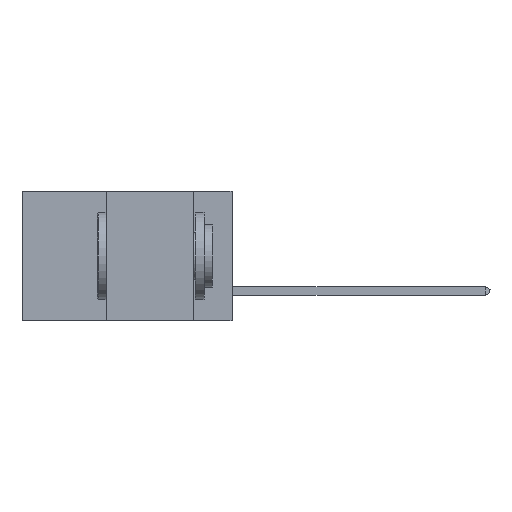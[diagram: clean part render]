
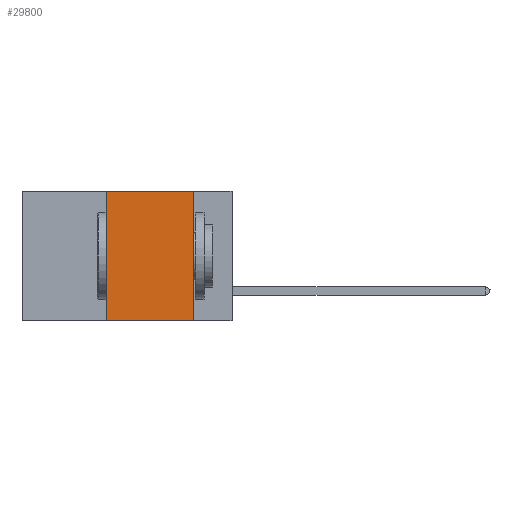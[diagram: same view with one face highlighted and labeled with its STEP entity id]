
A CAD part, left-side view. The second image highlights one B-rep face of the part: STEP entity #29800.
In plain terms, the highlighted planar face has unit normal (-1, 0, 0).
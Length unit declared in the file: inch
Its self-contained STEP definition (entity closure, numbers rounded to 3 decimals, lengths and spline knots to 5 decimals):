
#941 = LINE ( 'NONE', #6337, #48508 ) ;
#4822 = EDGE_CURVE ( 'NONE', #9141, #17668, #25303, .T. ) ;
#5923 = AXIS2_PLACEMENT_3D ( 'NONE', #14358, #9700, #25988 ) ;
#6009 = CARTESIAN_POINT ( 'NONE',  ( 0., 0.36, 0. ) ) ;
#6337 = CARTESIAN_POINT ( 'NONE',  ( 0., 0.6, -0.37 ) ) ;
#9141 = VERTEX_POINT ( 'NONE', #6009 ) ;
#9700 = DIRECTION ( 'NONE',  ( 1., 0., 0. ) ) ;
#13434 = EDGE_CURVE ( 'NONE', #17668, #29327, #38671, .T. ) ;
#14358 = CARTESIAN_POINT ( 'NONE',  ( 0., 0.6, 0. ) ) ;
#16142 = VECTOR ( 'NONE', #41430, 39.37008 ) ;
#17668 = VERTEX_POINT ( 'NONE', #37970 ) ;
#19001 = ORIENTED_EDGE ( 'NONE', *, *, #43399, .F. ) ;
#20560 = VECTOR ( 'NONE', #32418, 39.37008 ) ;
#24343 = VERTEX_POINT ( 'NONE', #46436 ) ;
#24676 = CARTESIAN_POINT ( 'NONE',  ( 0., 0.11, 0. ) ) ;
#25303 = LINE ( 'NONE', #40562, #16142 ) ;
#25525 = ORIENTED_EDGE ( 'NONE', *, *, #31946, .T. ) ;
#25988 = DIRECTION ( 'NONE',  ( 0., 0., -1. ) ) ;
#27235 = ORIENTED_EDGE ( 'NONE', *, *, #13434, .F. ) ;
#29327 = VERTEX_POINT ( 'NONE', #33696 ) ;
#29423 = DIRECTION ( 'NONE',  ( 0., -1., 0. ) ) ;
#29800 = ADVANCED_FACE ( 'NONE', ( #47466 ), #35439, .F. ) ;
#31506 = LINE ( 'NONE', #35094, #38179 ) ;
#31946 = EDGE_CURVE ( 'NONE', #24343, #29327, #941, .T. ) ;
#32418 = DIRECTION ( 'NONE',  ( 0., 0., -1. ) ) ;
#33696 = CARTESIAN_POINT ( 'NONE',  ( 0., 0.11, -0.37 ) ) ;
#35094 = CARTESIAN_POINT ( 'NONE',  ( 0., 0.36, 0. ) ) ;
#35439 = PLANE ( 'NONE',  #5923 ) ;
#37970 = CARTESIAN_POINT ( 'NONE',  ( 0., 0.11, 0. ) ) ;
#38179 = VECTOR ( 'NONE', #47461, 39.37008 ) ;
#38671 = LINE ( 'NONE', #24676, #20560 ) ;
#40562 = CARTESIAN_POINT ( 'NONE',  ( 0., 0.6, 0. ) ) ;
#41430 = DIRECTION ( 'NONE',  ( 0., -1., 0. ) ) ;
#43399 = EDGE_CURVE ( 'NONE', #24343, #9141, #31506, .T. ) ;
#43763 = ORIENTED_EDGE ( 'NONE', *, *, #4822, .F. ) ;
#44875 = EDGE_LOOP ( 'NONE', ( #27235, #43763, #19001, #25525 ) ) ;
#46436 = CARTESIAN_POINT ( 'NONE',  ( 0., 0.36, -0.37 ) ) ;
#47461 = DIRECTION ( 'NONE',  ( 0., 0., 1. ) ) ;
#47466 = FACE_OUTER_BOUND ( 'NONE', #44875, .T. ) ;
#48508 = VECTOR ( 'NONE', #29423, 39.37008 ) ;
